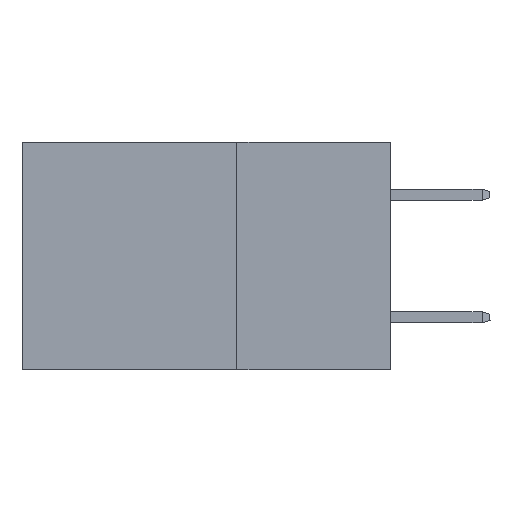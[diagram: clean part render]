
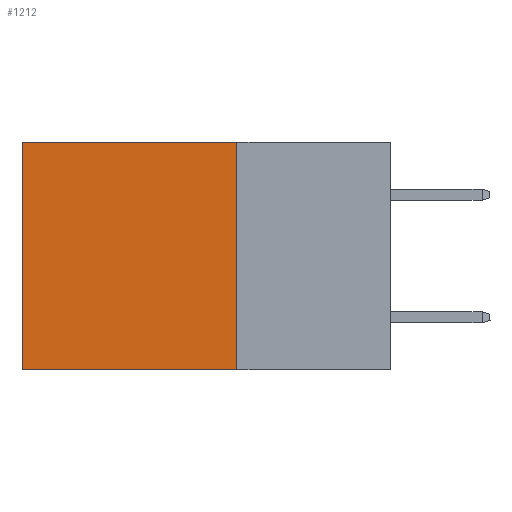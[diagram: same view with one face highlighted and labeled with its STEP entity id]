
A CAD part, left-side view. The second image highlights one B-rep face of the part: STEP entity #1212.
In plain terms, the highlighted planar face has unit normal (-1, 0, 0).
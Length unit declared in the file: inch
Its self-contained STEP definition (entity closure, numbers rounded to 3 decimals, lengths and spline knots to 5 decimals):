
#312 = VECTOR ( 'NONE', #3818, 39.37008 ) ;
#982 = ORIENTED_EDGE ( 'NONE', *, *, #10960, .T. ) ;
#1086 = LINE ( 'NONE', #8946, #9940 ) ;
#1212 = ADVANCED_FACE ( 'NONE', ( #13450 ), #9228, .F. ) ;
#1409 = LINE ( 'NONE', #5513, #10226 ) ;
#1482 = CARTESIAN_POINT ( 'NONE',  ( 0.2875, 0.6, -0.37 ) ) ;
#1484 = ORIENTED_EDGE ( 'NONE', *, *, #2871, .F. ) ;
#2709 = VERTEX_POINT ( 'NONE', #1482 ) ;
#2871 = EDGE_CURVE ( 'NONE', #12535, #2709, #1086, .T. ) ;
#3467 = LINE ( 'NONE', #13376, #9470 ) ;
#3507 = LINE ( 'NONE', #9778, #312 ) ;
#3818 = DIRECTION ( 'NONE',  ( 0., 0., -1. ) ) ;
#4142 = CARTESIAN_POINT ( 'NONE',  ( 0.2875, 0.25, -0.37 ) ) ;
#4998 = EDGE_CURVE ( 'NONE', #14641, #12535, #1409, .T. ) ;
#5512 = ORIENTED_EDGE ( 'NONE', *, *, #13045, .T. ) ;
#5513 = CARTESIAN_POINT ( 'NONE',  ( 0.2875, 0.25, 0. ) ) ;
#5600 = EDGE_LOOP ( 'NONE', ( #5512, #1484, #14352, #982 ) ) ;
#6460 = AXIS2_PLACEMENT_3D ( 'NONE', #9731, #9211, #9172 ) ;
#8946 = CARTESIAN_POINT ( 'NONE',  ( 0.2875, 0.25, -0.37 ) ) ;
#9172 = DIRECTION ( 'NONE',  ( 0., 0., -1. ) ) ;
#9211 = DIRECTION ( 'NONE',  ( 1., 0., 0. ) ) ;
#9228 = PLANE ( 'NONE',  #6460 ) ;
#9470 = VECTOR ( 'NONE', #14524, 39.37008 ) ;
#9731 = CARTESIAN_POINT ( 'NONE',  ( 0.2875, 0.25, 0. ) ) ;
#9778 = CARTESIAN_POINT ( 'NONE',  ( 0.2875, 0.6, 0. ) ) ;
#9940 = VECTOR ( 'NONE', #12488, 39.37008 ) ;
#10226 = VECTOR ( 'NONE', #13754, 39.37008 ) ;
#10960 = EDGE_CURVE ( 'NONE', #14641, #11218, #3467, .T. ) ;
#11218 = VERTEX_POINT ( 'NONE', #13466 ) ;
#12488 = DIRECTION ( 'NONE',  ( 0., 1., 0. ) ) ;
#12535 = VERTEX_POINT ( 'NONE', #4142 ) ;
#13045 = EDGE_CURVE ( 'NONE', #11218, #2709, #3507, .T. ) ;
#13376 = CARTESIAN_POINT ( 'NONE',  ( 0.2875, 0.25, 0. ) ) ;
#13450 = FACE_OUTER_BOUND ( 'NONE', #5600, .T. ) ;
#13466 = CARTESIAN_POINT ( 'NONE',  ( 0.2875, 0.6, 0. ) ) ;
#13754 = DIRECTION ( 'NONE',  ( 0., 0., -1. ) ) ;
#14024 = CARTESIAN_POINT ( 'NONE',  ( 0.2875, 0.25, 0. ) ) ;
#14352 = ORIENTED_EDGE ( 'NONE', *, *, #4998, .F. ) ;
#14524 = DIRECTION ( 'NONE',  ( 0., 1., 0. ) ) ;
#14641 = VERTEX_POINT ( 'NONE', #14024 ) ;
